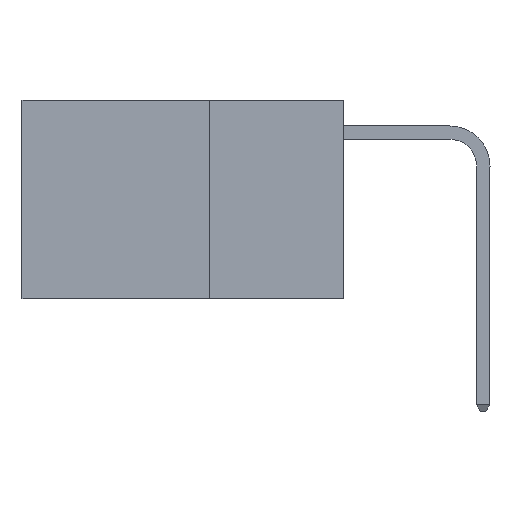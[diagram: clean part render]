
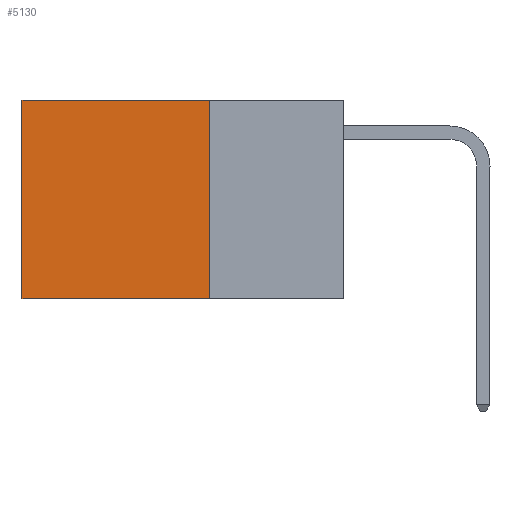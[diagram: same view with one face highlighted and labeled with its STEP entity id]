
A CAD part, left-side view. The second image highlights one B-rep face of the part: STEP entity #5130.
In plain terms, the highlighted planar face has unit normal (-1, 0, 0).
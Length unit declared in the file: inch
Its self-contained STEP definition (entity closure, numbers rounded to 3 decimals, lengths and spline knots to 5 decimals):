
#36 = CARTESIAN_POINT ( 'NONE',  ( 0.2625, 0.6, 0. ) ) ;
#321 = DIRECTION ( 'NONE',  ( 0., 0., -1. ) ) ;
#1341 = CARTESIAN_POINT ( 'NONE',  ( 0.2625, 0.25, 0. ) ) ;
#1441 = DIRECTION ( 'NONE',  ( 0., 1., 0. ) ) ;
#2177 = VERTEX_POINT ( 'NONE', #9969 ) ;
#3377 = PLANE ( 'NONE',  #3406 ) ;
#3406 = AXIS2_PLACEMENT_3D ( 'NONE', #3515, #3491, #3428 ) ;
#3428 = DIRECTION ( 'NONE',  ( 0., 0., -1. ) ) ;
#3491 = DIRECTION ( 'NONE',  ( 1., 0., 0. ) ) ;
#3515 = CARTESIAN_POINT ( 'NONE',  ( 0.2625, 0.25, 0. ) ) ;
#4082 = LINE ( 'NONE', #36, #4104 ) ;
#4104 = VECTOR ( 'NONE', #4854, 39.37008 ) ;
#4854 = DIRECTION ( 'NONE',  ( 0., 0., -1. ) ) ;
#4953 = VERTEX_POINT ( 'NONE', #6513 ) ;
#5051 = LINE ( 'NONE', #11196, #5350 ) ;
#5130 = ADVANCED_FACE ( 'NONE', ( #5219 ), #3377, .F. ) ;
#5219 = FACE_OUTER_BOUND ( 'NONE', #8510, .T. ) ;
#5350 = VECTOR ( 'NONE', #9448, 39.37008 ) ;
#5374 = VERTEX_POINT ( 'NONE', #11354 ) ;
#6128 = VERTEX_POINT ( 'NONE', #6133 ) ;
#6133 = CARTESIAN_POINT ( 'NONE',  ( 0.2625, 0.6, 0. ) ) ;
#6513 = CARTESIAN_POINT ( 'NONE',  ( 0.2625, 0.25, 0. ) ) ;
#7500 = EDGE_CURVE ( 'NONE', #4953, #6128, #8746, .T. ) ;
#8335 = ORIENTED_EDGE ( 'NONE', *, *, #11507, .F. ) ;
#8510 = EDGE_LOOP ( 'NONE', ( #9308, #8335, #11720, #9965 ) ) ;
#8700 = VECTOR ( 'NONE', #1441, 39.37008 ) ;
#8746 = LINE ( 'NONE', #1341, #8700 ) ;
#9308 = ORIENTED_EDGE ( 'NONE', *, *, #10481, .T. ) ;
#9448 = DIRECTION ( 'NONE',  ( 0., 1., 0. ) ) ;
#9965 = ORIENTED_EDGE ( 'NONE', *, *, #7500, .T. ) ;
#9969 = CARTESIAN_POINT ( 'NONE',  ( 0.2625, 0.25, -0.37 ) ) ;
#10481 = EDGE_CURVE ( 'NONE', #6128, #5374, #4082, .T. ) ;
#11196 = CARTESIAN_POINT ( 'NONE',  ( 0.2625, 0.25, -0.37 ) ) ;
#11354 = CARTESIAN_POINT ( 'NONE',  ( 0.2625, 0.6, -0.37 ) ) ;
#11430 = VECTOR ( 'NONE', #321, 39.37008 ) ;
#11507 = EDGE_CURVE ( 'NONE', #2177, #5374, #5051, .T. ) ;
#11694 = LINE ( 'NONE', #11763, #11430 ) ;
#11720 = ORIENTED_EDGE ( 'NONE', *, *, #11929, .F. ) ;
#11763 = CARTESIAN_POINT ( 'NONE',  ( 0.2625, 0.25, 0. ) ) ;
#11929 = EDGE_CURVE ( 'NONE', #4953, #2177, #11694, .T. ) ;
